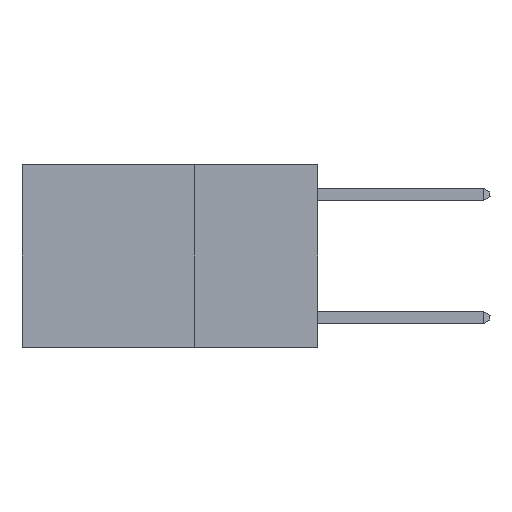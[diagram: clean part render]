
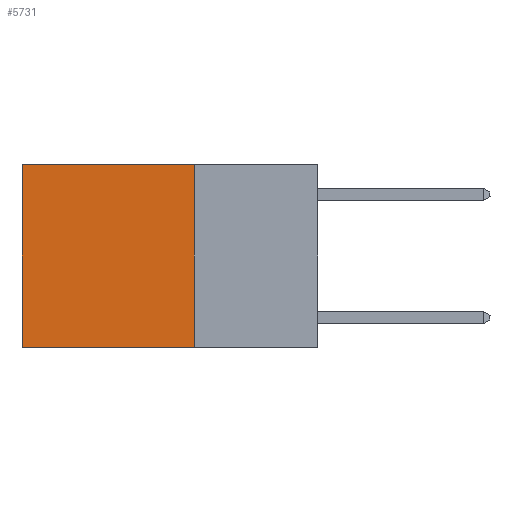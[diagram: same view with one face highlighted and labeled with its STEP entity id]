
A CAD part, left-side view. The second image highlights one B-rep face of the part: STEP entity #5731.
In plain terms, the highlighted planar face has unit normal (-1, 0, 0).
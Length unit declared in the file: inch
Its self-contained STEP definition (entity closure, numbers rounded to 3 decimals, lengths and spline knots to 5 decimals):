
#57 = VERTEX_POINT ( 'NONE', #9317 ) ;
#505 = DIRECTION ( 'NONE',  ( 1., 0., 0. ) ) ;
#590 = CARTESIAN_POINT ( 'NONE',  ( 0.2625, 0.25, 0. ) ) ;
#709 = EDGE_CURVE ( 'NONE', #15619, #866, #1193, .T. ) ;
#740 = DIRECTION ( 'NONE',  ( 0., 1., 0. ) ) ;
#825 = EDGE_LOOP ( 'NONE', ( #9898, #9267, #890, #4854 ) ) ;
#866 = VERTEX_POINT ( 'NONE', #6599 ) ;
#890 = ORIENTED_EDGE ( 'NONE', *, *, #709, .F. ) ;
#1193 = LINE ( 'NONE', #7323, #14428 ) ;
#1370 = LINE ( 'NONE', #13386, #2519 ) ;
#1715 = VECTOR ( 'NONE', #15494, 39.37008 ) ;
#2015 = CARTESIAN_POINT ( 'NONE',  ( 0.2625, 0.6, 0. ) ) ;
#2346 = DIRECTION ( 'NONE',  ( 0., 1., 0. ) ) ;
#2519 = VECTOR ( 'NONE', #2346, 39.37008 ) ;
#4329 = DIRECTION ( 'NONE',  ( 0., 0., -1. ) ) ;
#4581 = VERTEX_POINT ( 'NONE', #8030 ) ;
#4854 = ORIENTED_EDGE ( 'NONE', *, *, #7716, .T. ) ;
#5731 = ADVANCED_FACE ( 'NONE', ( #11639 ), #11556, .F. ) ;
#6007 = CARTESIAN_POINT ( 'NONE',  ( 0.2625, 0.25, 0. ) ) ;
#6599 = CARTESIAN_POINT ( 'NONE',  ( 0.2625, 0.25, -0.37 ) ) ;
#7323 = CARTESIAN_POINT ( 'NONE',  ( 0.2625, 0.25, 0. ) ) ;
#7488 = DIRECTION ( 'NONE',  ( 0., 0., -1. ) ) ;
#7716 = EDGE_CURVE ( 'NONE', #15619, #4581, #10881, .T. ) ;
#7913 = EDGE_CURVE ( 'NONE', #866, #57, #1370, .T. ) ;
#8030 = CARTESIAN_POINT ( 'NONE',  ( 0.2625, 0.6, 0. ) ) ;
#9267 = ORIENTED_EDGE ( 'NONE', *, *, #7913, .F. ) ;
#9317 = CARTESIAN_POINT ( 'NONE',  ( 0.2625, 0.6, -0.37 ) ) ;
#9898 = ORIENTED_EDGE ( 'NONE', *, *, #15520, .T. ) ;
#10491 = LINE ( 'NONE', #2015, #1715 ) ;
#10881 = LINE ( 'NONE', #11789, #14106 ) ;
#11556 = PLANE ( 'NONE',  #12165 ) ;
#11639 = FACE_OUTER_BOUND ( 'NONE', #825, .T. ) ;
#11789 = CARTESIAN_POINT ( 'NONE',  ( 0.2625, 0.25, 0. ) ) ;
#12165 = AXIS2_PLACEMENT_3D ( 'NONE', #590, #505, #4329 ) ;
#13386 = CARTESIAN_POINT ( 'NONE',  ( 0.2625, 0.25, -0.37 ) ) ;
#14106 = VECTOR ( 'NONE', #740, 39.37008 ) ;
#14428 = VECTOR ( 'NONE', #7488, 39.37008 ) ;
#15494 = DIRECTION ( 'NONE',  ( 0., 0., -1. ) ) ;
#15520 = EDGE_CURVE ( 'NONE', #4581, #57, #10491, .T. ) ;
#15619 = VERTEX_POINT ( 'NONE', #6007 ) ;
